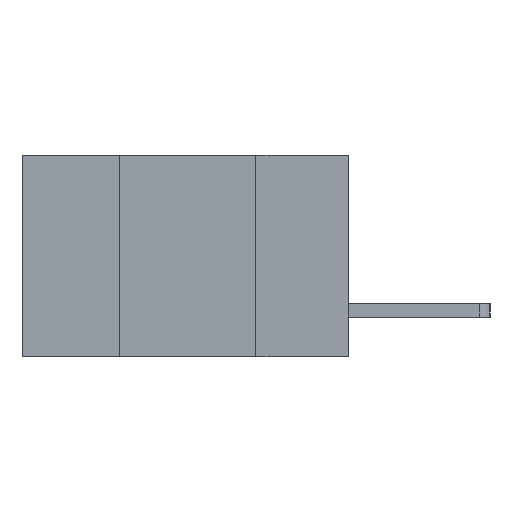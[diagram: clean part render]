
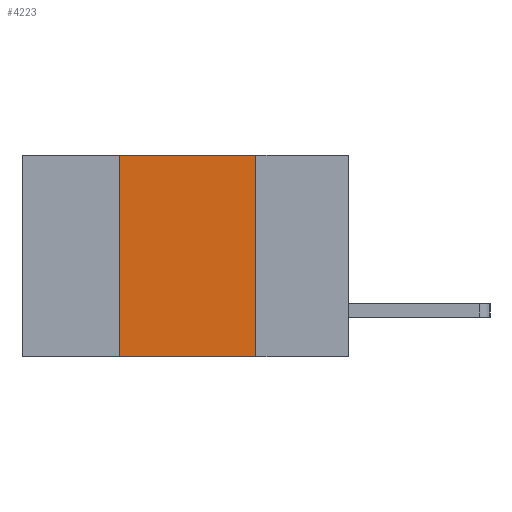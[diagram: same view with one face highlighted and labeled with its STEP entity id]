
A CAD part, left-side view. The second image highlights one B-rep face of the part: STEP entity #4223.
In plain terms, the highlighted planar face has unit normal (-1, 0, 0).
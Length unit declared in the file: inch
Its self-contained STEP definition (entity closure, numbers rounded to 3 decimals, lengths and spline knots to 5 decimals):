
#143 = PLANE ( 'NONE',  #7683 ) ;
#312 = VERTEX_POINT ( 'NONE', #9057 ) ;
#331 = CARTESIAN_POINT ( 'NONE',  ( 0., 0.6, 0. ) ) ;
#610 = FACE_OUTER_BOUND ( 'NONE', #5655, .T. ) ;
#719 = VECTOR ( 'NONE', #2601, 39.37008 ) ;
#877 = ORIENTED_EDGE ( 'NONE', *, *, #1251, .F. ) ;
#1182 = LINE ( 'NONE', #331, #719 ) ;
#1251 = EDGE_CURVE ( 'NONE', #312, #6412, #7495, .T. ) ;
#1495 = EDGE_CURVE ( 'NONE', #6677, #6412, #9336, .T. ) ;
#1570 = CARTESIAN_POINT ( 'NONE',  ( 0., 0.17, -0.37 ) ) ;
#1703 = VECTOR ( 'NONE', #7772, 39.37008 ) ;
#2601 = DIRECTION ( 'NONE',  ( 0., -1., 0. ) ) ;
#2928 = CARTESIAN_POINT ( 'NONE',  ( 0., 0.42, -0.37 ) ) ;
#3261 = ORIENTED_EDGE ( 'NONE', *, *, #9253, .F. ) ;
#3329 = LINE ( 'NONE', #9003, #9000 ) ;
#3341 = CARTESIAN_POINT ( 'NONE',  ( 0., 0.6, -0.37 ) ) ;
#3816 = ORIENTED_EDGE ( 'NONE', *, *, #5104, .F. ) ;
#3828 = DIRECTION ( 'NONE',  ( 0., 0., 1. ) ) ;
#3872 = DIRECTION ( 'NONE',  ( 0., 0., -1. ) ) ;
#4223 = ADVANCED_FACE ( 'NONE', ( #610 ), #143, .F. ) ;
#4517 = CARTESIAN_POINT ( 'NONE',  ( 0., 0.42, 0. ) ) ;
#5104 = EDGE_CURVE ( 'NONE', #7409, #312, #1182, .T. ) ;
#5525 = VECTOR ( 'NONE', #7489, 39.37008 ) ;
#5655 = EDGE_LOOP ( 'NONE', ( #877, #3816, #3261, #9455 ) ) ;
#6412 = VERTEX_POINT ( 'NONE', #8533 ) ;
#6677 = VERTEX_POINT ( 'NONE', #2928 ) ;
#6809 = CARTESIAN_POINT ( 'NONE',  ( 0., 0.6, 0. ) ) ;
#7409 = VERTEX_POINT ( 'NONE', #4517 ) ;
#7489 = DIRECTION ( 'NONE',  ( 0., 0., -1. ) ) ;
#7495 = LINE ( 'NONE', #1570, #5525 ) ;
#7683 = AXIS2_PLACEMENT_3D ( 'NONE', #6809, #8320, #3872 ) ;
#7772 = DIRECTION ( 'NONE',  ( 0., -1., 0. ) ) ;
#8320 = DIRECTION ( 'NONE',  ( 1., 0., 0. ) ) ;
#8533 = CARTESIAN_POINT ( 'NONE',  ( 0., 0.17, -0.37 ) ) ;
#9000 = VECTOR ( 'NONE', #3828, 39.37008 ) ;
#9003 = CARTESIAN_POINT ( 'NONE',  ( 0., 0.42, -0.37 ) ) ;
#9057 = CARTESIAN_POINT ( 'NONE',  ( 0., 0.17, 0. ) ) ;
#9253 = EDGE_CURVE ( 'NONE', #6677, #7409, #3329, .T. ) ;
#9336 = LINE ( 'NONE', #3341, #1703 ) ;
#9455 = ORIENTED_EDGE ( 'NONE', *, *, #1495, .T. ) ;
